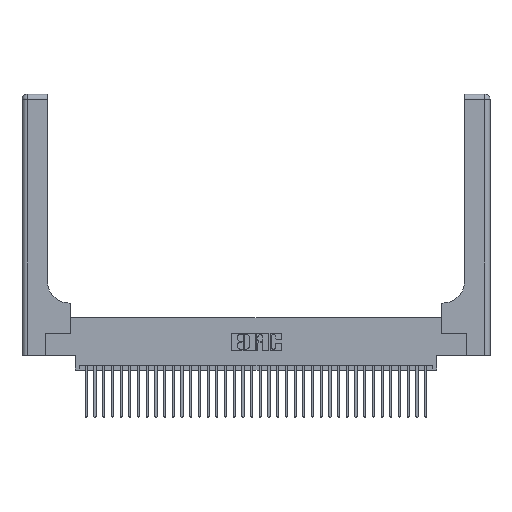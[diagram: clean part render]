
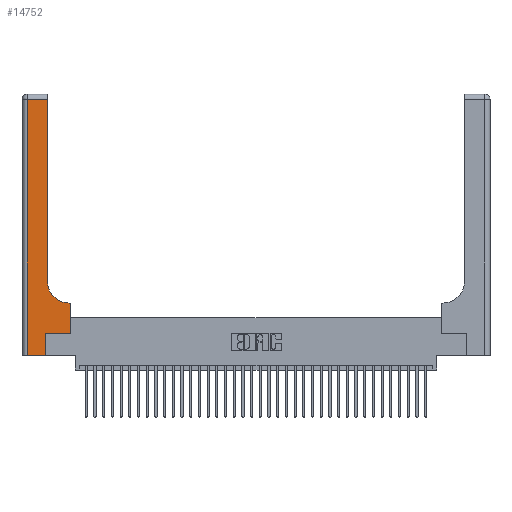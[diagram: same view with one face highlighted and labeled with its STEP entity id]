
A CAD part, top view. The second image highlights one B-rep face of the part: STEP entity #14752.
In plain terms, the highlighted planar face has unit normal (0, 0, 1).
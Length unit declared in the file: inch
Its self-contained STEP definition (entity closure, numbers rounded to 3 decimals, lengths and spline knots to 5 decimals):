
#2957 = ORIENTED_EDGE ( 'NONE', *, *, #27647, .T. ) ;
#3685 = VECTOR ( 'NONE', #31308, 39.37008 ) ;
#3768 = CARTESIAN_POINT ( 'NONE',  ( 0., 2.94, 0.37 ) ) ;
#4842 = ORIENTED_EDGE ( 'NONE', *, *, #29622, .T. ) ;
#5218 = DIRECTION ( 'NONE',  ( 0., 0., -1. ) ) ;
#5445 = CARTESIAN_POINT ( 'NONE',  ( 0.5585, 0.6, 0.37 ) ) ;
#5849 = EDGE_CURVE ( 'NONE', #27878, #18899, #22136, .T. ) ;
#6094 = VECTOR ( 'NONE', #23995, 39.37008 ) ;
#6499 = LINE ( 'NONE', #8221, #12811 ) ;
#7851 = VECTOR ( 'NONE', #20411, 39.37008 ) ;
#8098 = CARTESIAN_POINT ( 'NONE',  ( 0., 3., 0.37 ) ) ;
#8221 = CARTESIAN_POINT ( 'NONE',  ( 0.2915, 0.6, 0.37 ) ) ;
#10117 = VECTOR ( 'NONE', #12232, 39.37008 ) ;
#10453 = EDGE_CURVE ( 'NONE', #29785, #10699, #18080, .T. ) ;
#10699 = VERTEX_POINT ( 'NONE', #21729 ) ;
#10788 = CARTESIAN_POINT ( 'NONE',  ( 0.06, 3., 0.37 ) ) ;
#10981 = DIRECTION ( 'NONE',  ( -1., 0., 0. ) ) ;
#11357 = CARTESIAN_POINT ( 'NONE',  ( 0.5415, 0.6, 0.37 ) ) ;
#11494 = CARTESIAN_POINT ( 'NONE',  ( 0., 0., 0.37 ) ) ;
#11534 = ORIENTED_EDGE ( 'NONE', *, *, #23357, .T. ) ;
#11537 = VERTEX_POINT ( 'NONE', #24532 ) ;
#11560 = VECTOR ( 'NONE', #14563, 39.37008 ) ;
#11838 = CARTESIAN_POINT ( 'NONE',  ( 0.269, 0., 0.37 ) ) ;
#12232 = DIRECTION ( 'NONE',  ( 1., 0., 0. ) ) ;
#12552 = CARTESIAN_POINT ( 'NONE',  ( 0.5415, 0.85, 0.37 ) ) ;
#12754 = ORIENTED_EDGE ( 'NONE', *, *, #34112, .T. ) ;
#12811 = VECTOR ( 'NONE', #19799, 39.37008 ) ;
#12813 = DIRECTION ( 'NONE',  ( 0., 0., -1. ) ) ;
#12967 = LINE ( 'NONE', #10788, #29487 ) ;
#13465 = CARTESIAN_POINT ( 'NONE',  ( 0.06, 0., 0.37 ) ) ;
#14339 = VECTOR ( 'NONE', #23012, 39.37008 ) ;
#14563 = DIRECTION ( 'NONE',  ( 0., 1., 0. ) ) ;
#14752 = ADVANCED_FACE ( 'NONE', ( #26628 ), #25052, .F. ) ;
#15248 = CARTESIAN_POINT ( 'NONE',  ( 0.2915, 2.94, 0.37 ) ) ;
#15648 = DIRECTION ( 'NONE',  ( 1., 0., 0. ) ) ;
#16715 = ORIENTED_EDGE ( 'NONE', *, *, #34483, .T. ) ;
#17182 = CARTESIAN_POINT ( 'NONE',  ( 0.2915, 3., 0.37 ) ) ;
#17425 = EDGE_CURVE ( 'NONE', #34666, #11537, #31843, .T. ) ;
#17655 = LINE ( 'NONE', #26345, #10117 ) ;
#18045 = ORIENTED_EDGE ( 'NONE', *, *, #17425, .T. ) ;
#18080 = LINE ( 'NONE', #3768, #6094 ) ;
#18899 = VERTEX_POINT ( 'NONE', #20055 ) ;
#19799 = DIRECTION ( 'NONE',  ( -1., 0., 0. ) ) ;
#20055 = CARTESIAN_POINT ( 'NONE',  ( 0.2915, 0.85, 0.37 ) ) ;
#20411 = DIRECTION ( 'NONE',  ( 1., 0., 0. ) ) ;
#21729 = CARTESIAN_POINT ( 'NONE',  ( 0.06, 2.94, 0.37 ) ) ;
#22136 = CIRCLE ( 'NONE', #24048, 0.25 ) ;
#22673 = EDGE_LOOP ( 'NONE', ( #2957, #33119, #16715, #4842, #18045, #11534, #12754, #30523, #26842 ) ) ;
#22988 = EDGE_CURVE ( 'NONE', #28886, #27878, #6499, .T. ) ;
#23012 = DIRECTION ( 'NONE',  ( 0., 1., 0. ) ) ;
#23357 = EDGE_CURVE ( 'NONE', #11537, #28543, #17655, .T. ) ;
#23995 = DIRECTION ( 'NONE',  ( -1., 0., 0. ) ) ;
#23996 = LINE ( 'NONE', #17182, #11560 ) ;
#24048 = AXIS2_PLACEMENT_3D ( 'NONE', #12552, #12813, #15648 ) ;
#24532 = CARTESIAN_POINT ( 'NONE',  ( 0.269, 0.25, 0.37 ) ) ;
#25052 = PLANE ( 'NONE',  #33314 ) ;
#25490 = VERTEX_POINT ( 'NONE', #13465 ) ;
#25766 = CARTESIAN_POINT ( 'NONE',  ( 0.5585, 0.25, 0.37 ) ) ;
#26093 = LINE ( 'NONE', #11494, #7851 ) ;
#26345 = CARTESIAN_POINT ( 'NONE',  ( 0.269, 0.25, 0.37 ) ) ;
#26628 = FACE_OUTER_BOUND ( 'NONE', #22673, .T. ) ;
#26842 = ORIENTED_EDGE ( 'NONE', *, *, #5849, .T. ) ;
#27647 = EDGE_CURVE ( 'NONE', #18899, #29785, #23996, .T. ) ;
#27878 = VERTEX_POINT ( 'NONE', #11357 ) ;
#28100 = CARTESIAN_POINT ( 'NONE',  ( 0.269, 0., 0.37 ) ) ;
#28543 = VERTEX_POINT ( 'NONE', #35099 ) ;
#28886 = VERTEX_POINT ( 'NONE', #5445 ) ;
#29487 = VECTOR ( 'NONE', #30835, 39.37008 ) ;
#29622 = EDGE_CURVE ( 'NONE', #25490, #34666, #26093, .T. ) ;
#29785 = VERTEX_POINT ( 'NONE', #15248 ) ;
#29947 = LINE ( 'NONE', #25766, #14339 ) ;
#30523 = ORIENTED_EDGE ( 'NONE', *, *, #22988, .T. ) ;
#30835 = DIRECTION ( 'NONE',  ( 0., -1., 0. ) ) ;
#31308 = DIRECTION ( 'NONE',  ( 0., 1., 0. ) ) ;
#31843 = LINE ( 'NONE', #28100, #3685 ) ;
#33119 = ORIENTED_EDGE ( 'NONE', *, *, #10453, .T. ) ;
#33314 = AXIS2_PLACEMENT_3D ( 'NONE', #8098, #5218, #10981 ) ;
#34112 = EDGE_CURVE ( 'NONE', #28543, #28886, #29947, .T. ) ;
#34483 = EDGE_CURVE ( 'NONE', #10699, #25490, #12967, .T. ) ;
#34666 = VERTEX_POINT ( 'NONE', #11838 ) ;
#35099 = CARTESIAN_POINT ( 'NONE',  ( 0.5585, 0.25, 0.37 ) ) ;
